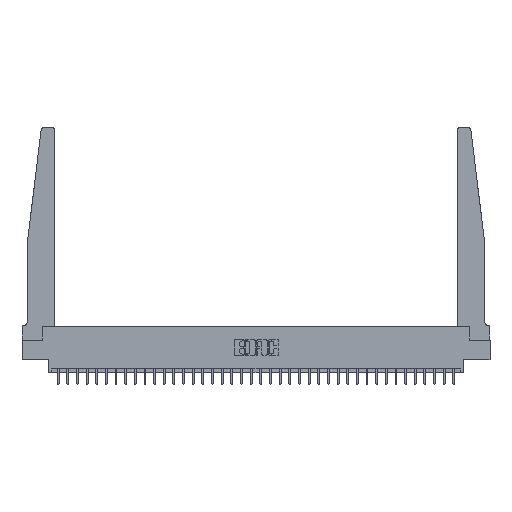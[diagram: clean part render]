
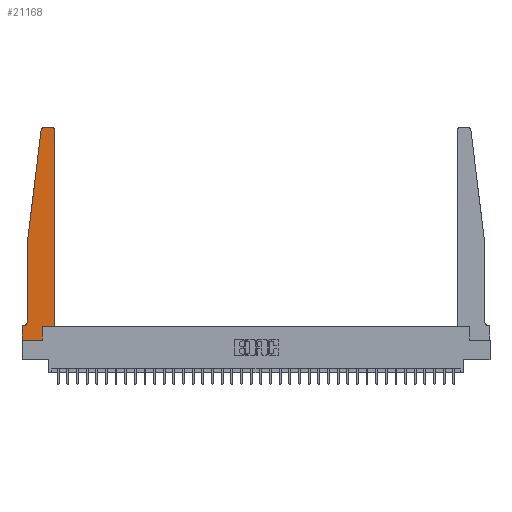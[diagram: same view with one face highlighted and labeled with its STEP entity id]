
A CAD part, top view. The second image highlights one B-rep face of the part: STEP entity #21168.
In plain terms, the highlighted planar face has unit normal (0, 0, 1).
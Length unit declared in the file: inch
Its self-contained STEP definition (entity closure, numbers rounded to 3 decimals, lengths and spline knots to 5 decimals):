
#632 = VERTEX_POINT ( 'NONE', #14796 ) ;
#901 = VERTEX_POINT ( 'NONE', #10560 ) ;
#1013 = EDGE_CURVE ( 'NONE', #30411, #20433, #31781, .T. ) ;
#1621 = CARTESIAN_POINT ( 'NONE',  ( 0.25, 2.75, 0.37 ) ) ;
#2290 = CARTESIAN_POINT ( 'NONE',  ( 0.27653, 2.75, 0.37 ) ) ;
#2501 = CARTESIAN_POINT ( 'NONE',  ( 0.2605, 0.18, 0.37 ) ) ;
#2741 = CIRCLE ( 'NONE', #30826, 0.05 ) ;
#2859 = ORIENTED_EDGE ( 'NONE', *, *, #19825, .T. ) ;
#4137 = LINE ( 'NONE', #13327, #22420 ) ;
#4507 = EDGE_CURVE ( 'NONE', #11505, #14677, #20461, .T. ) ;
#4922 = ORIENTED_EDGE ( 'NONE', *, *, #4507, .T. ) ;
#5909 = CARTESIAN_POINT ( 'NONE',  ( 0., 0.1875, 0.37 ) ) ;
#6056 = VECTOR ( 'NONE', #13929, 39.37008 ) ;
#6709 = DIRECTION ( 'NONE',  ( 0., 0., 1. ) ) ;
#6878 = DIRECTION ( 'NONE',  ( 1., 0., 0. ) ) ;
#7323 = CARTESIAN_POINT ( 'NONE',  ( 0.395, 2.72, 0.37 ) ) ;
#7391 = EDGE_CURVE ( 'NONE', #901, #10331, #19200, .T. ) ;
#7539 = VERTEX_POINT ( 'NONE', #15535 ) ;
#7597 = VECTOR ( 'NONE', #30579, 39.37008 ) ;
#8812 = LINE ( 'NONE', #18904, #6056 ) ;
#9013 = CARTESIAN_POINT ( 'NONE',  ( 0.065, 1.25, 0.37 ) ) ;
#9157 = VERTEX_POINT ( 'NONE', #9013 ) ;
#10200 = ORIENTED_EDGE ( 'NONE', *, *, #24779, .T. ) ;
#10331 = VERTEX_POINT ( 'NONE', #5909 ) ;
#10560 = CARTESIAN_POINT ( 'NONE',  ( 0.015, 0.1875, 0.37 ) ) ;
#10668 = ORIENTED_EDGE ( 'NONE', *, *, #1013, .T. ) ;
#10857 = LINE ( 'NONE', #25786, #7597 ) ;
#11078 = DIRECTION ( 'NONE',  ( 0., 0., -1. ) ) ;
#11142 = ORIENTED_EDGE ( 'NONE', *, *, #14605, .T. ) ;
#11218 = VECTOR ( 'NONE', #14894, 39.37008 ) ;
#11320 = LINE ( 'NONE', #18786, #31948 ) ;
#11505 = VERTEX_POINT ( 'NONE', #15036 ) ;
#11561 = DIRECTION ( 'NONE',  ( 0., 0., 1. ) ) ;
#11684 = ORIENTED_EDGE ( 'NONE', *, *, #25441, .T. ) ;
#13122 = AXIS2_PLACEMENT_3D ( 'NONE', #7323, #27061, #27384 ) ;
#13182 = DIRECTION ( 'NONE',  ( 0., 1., 0. ) ) ;
#13324 = ORIENTED_EDGE ( 'NONE', *, *, #25987, .T. ) ;
#13327 = CARTESIAN_POINT ( 'NONE',  ( 0., 0., 0.37 ) ) ;
#13397 = ORIENTED_EDGE ( 'NONE', *, *, #7391, .T. ) ;
#13929 = DIRECTION ( 'NONE',  ( 0., 1., 0. ) ) ;
#14042 = FACE_OUTER_BOUND ( 'NONE', #25501, .T. ) ;
#14257 = CIRCLE ( 'NONE', #13122, 0.03 ) ;
#14605 = EDGE_CURVE ( 'NONE', #26897, #23154, #14257, .T. ) ;
#14677 = VERTEX_POINT ( 'NONE', #2501 ) ;
#14796 = CARTESIAN_POINT ( 'NONE',  ( 0.065, 0.2375, 0.37 ) ) ;
#14894 = DIRECTION ( 'NONE',  ( 0., -1., 0. ) ) ;
#15036 = CARTESIAN_POINT ( 'NONE',  ( 0.2605, 0., 0.37 ) ) ;
#15132 = ORIENTED_EDGE ( 'NONE', *, *, #28128, .T. ) ;
#15535 = CARTESIAN_POINT ( 'NONE',  ( 0.425, 0.18, 0.37 ) ) ;
#15718 = DIRECTION ( 'NONE',  ( -1., 0., 0. ) ) ;
#16523 = ORIENTED_EDGE ( 'NONE', *, *, #22482, .T. ) ;
#17064 = DIRECTION ( 'NONE',  ( 1., 0., 0. ) ) ;
#17162 = CARTESIAN_POINT ( 'NONE',  ( 0.425, 2.72, 0.37 ) ) ;
#18786 = CARTESIAN_POINT ( 'NONE',  ( 0.425, 0.18, 0.37 ) ) ;
#18904 = CARTESIAN_POINT ( 'NONE',  ( 0.425, 0.18, 0.37 ) ) ;
#19200 = LINE ( 'NONE', #22023, #25984 ) ;
#19688 = LINE ( 'NONE', #1621, #22971 ) ;
#19749 = EDGE_CURVE ( 'NONE', #10331, #26525, #20354, .T. ) ;
#19825 = EDGE_CURVE ( 'NONE', #632, #901, #2741, .T. ) ;
#20354 = LINE ( 'NONE', #29837, #11218 ) ;
#20433 = VERTEX_POINT ( 'NONE', #25071 ) ;
#20461 = LINE ( 'NONE', #28109, #28245 ) ;
#21168 = ADVANCED_FACE ( 'NONE', ( #14042 ), #24002, .T. ) ;
#21680 = DIRECTION ( 'NONE',  ( 1., 0., 0. ) ) ;
#22023 = CARTESIAN_POINT ( 'NONE',  ( 0.065, 0.1875, 0.37 ) ) ;
#22173 = LINE ( 'NONE', #22495, #29808 ) ;
#22420 = VECTOR ( 'NONE', #17064, 39.37008 ) ;
#22482 = EDGE_CURVE ( 'NONE', #9157, #632, #22173, .T. ) ;
#22495 = CARTESIAN_POINT ( 'NONE',  ( 0.065, 1.25, 0.37 ) ) ;
#22971 = VECTOR ( 'NONE', #29817, 39.37008 ) ;
#23154 = VERTEX_POINT ( 'NONE', #32159 ) ;
#23256 = EDGE_CURVE ( 'NONE', #26525, #11505, #4137, .T. ) ;
#24002 = PLANE ( 'NONE',  #29835 ) ;
#24503 = CARTESIAN_POINT ( 'NONE',  ( 0., 0.1875, 0.37 ) ) ;
#24779 = EDGE_CURVE ( 'NONE', #7539, #26897, #8812, .T. ) ;
#25071 = CARTESIAN_POINT ( 'NONE',  ( 0.24675, 2.72367, 0.37 ) ) ;
#25441 = EDGE_CURVE ( 'NONE', #20433, #9157, #10857, .T. ) ;
#25445 = AXIS2_PLACEMENT_3D ( 'NONE', #29609, #6709, #6878 ) ;
#25501 = EDGE_LOOP ( 'NONE', ( #15132, #10668, #11684, #16523, #2859, #13397, #30883, #29877, #4922, #13324, #10200, #11142 ) ) ;
#25786 = CARTESIAN_POINT ( 'NONE',  ( 0.065, 1.25, 0.37 ) ) ;
#25984 = VECTOR ( 'NONE', #31974, 39.37008 ) ;
#25987 = EDGE_CURVE ( 'NONE', #14677, #7539, #11320, .T. ) ;
#26429 = DIRECTION ( 'NONE',  ( 1., 0., 0. ) ) ;
#26525 = VERTEX_POINT ( 'NONE', #30333 ) ;
#26897 = VERTEX_POINT ( 'NONE', #17162 ) ;
#27061 = DIRECTION ( 'NONE',  ( 0., 0., 1. ) ) ;
#27384 = DIRECTION ( 'NONE',  ( 1., 0., 0. ) ) ;
#28109 = CARTESIAN_POINT ( 'NONE',  ( 0.2605, 0.18, 0.37 ) ) ;
#28128 = EDGE_CURVE ( 'NONE', #23154, #30411, #19688, .T. ) ;
#28245 = VECTOR ( 'NONE', #13182, 39.37008 ) ;
#29609 = CARTESIAN_POINT ( 'NONE',  ( 0.27653, 2.72, 0.37 ) ) ;
#29808 = VECTOR ( 'NONE', #32610, 39.37008 ) ;
#29817 = DIRECTION ( 'NONE',  ( -1., 0., 0. ) ) ;
#29835 = AXIS2_PLACEMENT_3D ( 'NONE', #24503, #11561, #21680 ) ;
#29837 = CARTESIAN_POINT ( 'NONE',  ( 0., 0., 0.37 ) ) ;
#29877 = ORIENTED_EDGE ( 'NONE', *, *, #23256, .T. ) ;
#30333 = CARTESIAN_POINT ( 'NONE',  ( 0., 0., 0.37 ) ) ;
#30411 = VERTEX_POINT ( 'NONE', #2290 ) ;
#30579 = DIRECTION ( 'NONE',  ( -0.122, -0.992, 0. ) ) ;
#30826 = AXIS2_PLACEMENT_3D ( 'NONE', #31145, #11078, #15718 ) ;
#30883 = ORIENTED_EDGE ( 'NONE', *, *, #19749, .T. ) ;
#31145 = CARTESIAN_POINT ( 'NONE',  ( 0.015, 0.2375, 0.37 ) ) ;
#31781 = CIRCLE ( 'NONE', #25445, 0.03 ) ;
#31948 = VECTOR ( 'NONE', #26429, 39.37008 ) ;
#31974 = DIRECTION ( 'NONE',  ( -1., 0., 0. ) ) ;
#32159 = CARTESIAN_POINT ( 'NONE',  ( 0.395, 2.75, 0.37 ) ) ;
#32610 = DIRECTION ( 'NONE',  ( 0., -1., 0. ) ) ;
